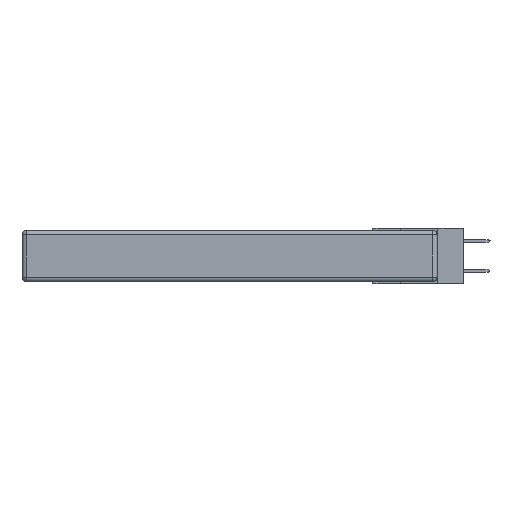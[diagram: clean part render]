
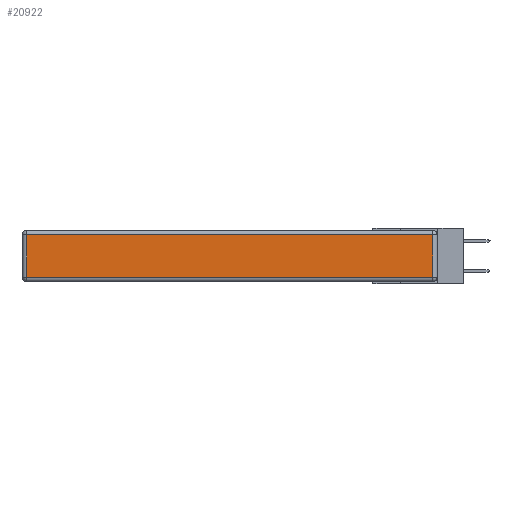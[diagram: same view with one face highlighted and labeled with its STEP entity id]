
A CAD part, left-side view. The second image highlights one B-rep face of the part: STEP entity #20922.
In plain terms, the highlighted planar face has unit normal (-1, 0, 0).
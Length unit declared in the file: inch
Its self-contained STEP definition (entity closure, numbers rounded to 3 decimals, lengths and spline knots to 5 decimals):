
#1873 = EDGE_LOOP ( 'NONE', ( #19638, #11738, #25338, #19341 ) ) ;
#1945 = LINE ( 'NONE', #6239, #19402 ) ;
#2250 = LINE ( 'NONE', #6482, #4998 ) ;
#2380 = LINE ( 'NONE', #18816, #21531 ) ;
#2396 = DIRECTION ( 'NONE',  ( 0., 0., 1. ) ) ;
#2602 = VERTEX_POINT ( 'NONE', #20364 ) ;
#4606 = CARTESIAN_POINT ( 'NONE',  ( 0., 0., -0.343 ) ) ;
#4807 = CARTESIAN_POINT ( 'NONE',  ( 0., 2.72, -0.03 ) ) ;
#4998 = VECTOR ( 'NONE', #26303, 39.37008 ) ;
#5048 = CARTESIAN_POINT ( 'NONE',  ( 0., 2.75, -0.03 ) ) ;
#6008 = EDGE_CURVE ( 'NONE', #15277, #22366, #1945, .T. ) ;
#6239 = CARTESIAN_POINT ( 'NONE',  ( 0., 2.72, -0.343 ) ) ;
#6482 = CARTESIAN_POINT ( 'NONE',  ( 0., 0.03, -0.343 ) ) ;
#8782 = FACE_OUTER_BOUND ( 'NONE', #1873, .T. ) ;
#9635 = DIRECTION ( 'NONE',  ( 0., 1., 0. ) ) ;
#10376 = VERTEX_POINT ( 'NONE', #20530 ) ;
#11205 = DIRECTION ( 'NONE',  ( -1., 0., 0. ) ) ;
#11738 = ORIENTED_EDGE ( 'NONE', *, *, #25888, .T. ) ;
#15277 = VERTEX_POINT ( 'NONE', #4807 ) ;
#15497 = CARTESIAN_POINT ( 'NONE',  ( 0., 2.72, -0.313 ) ) ;
#16520 = DIRECTION ( 'NONE',  ( 0., -1., 0. ) ) ;
#18816 = CARTESIAN_POINT ( 'NONE',  ( 0., 0., -0.313 ) ) ;
#19341 = ORIENTED_EDGE ( 'NONE', *, *, #6008, .T. ) ;
#19402 = VECTOR ( 'NONE', #26147, 39.37008 ) ;
#19638 = ORIENTED_EDGE ( 'NONE', *, *, #27003, .T. ) ;
#20364 = CARTESIAN_POINT ( 'NONE',  ( 0., 0.03, -0.313 ) ) ;
#20530 = CARTESIAN_POINT ( 'NONE',  ( 0., 0.03, -0.03 ) ) ;
#20922 = ADVANCED_FACE ( 'NONE', ( #8782 ), #26370, .T. ) ;
#21421 = VECTOR ( 'NONE', #9635, 39.37008 ) ;
#21531 = VECTOR ( 'NONE', #16520, 39.37008 ) ;
#22366 = VERTEX_POINT ( 'NONE', #15497 ) ;
#22800 = LINE ( 'NONE', #5048, #21421 ) ;
#25338 = ORIENTED_EDGE ( 'NONE', *, *, #25513, .T. ) ;
#25513 = EDGE_CURVE ( 'NONE', #10376, #15277, #22800, .T. ) ;
#25888 = EDGE_CURVE ( 'NONE', #2602, #10376, #2250, .T. ) ;
#26147 = DIRECTION ( 'NONE',  ( 0., 0., -1. ) ) ;
#26303 = DIRECTION ( 'NONE',  ( 0., 0., 1. ) ) ;
#26370 = PLANE ( 'NONE',  #26814 ) ;
#26814 = AXIS2_PLACEMENT_3D ( 'NONE', #4606, #11205, #2396 ) ;
#27003 = EDGE_CURVE ( 'NONE', #22366, #2602, #2380, .T. ) ;
